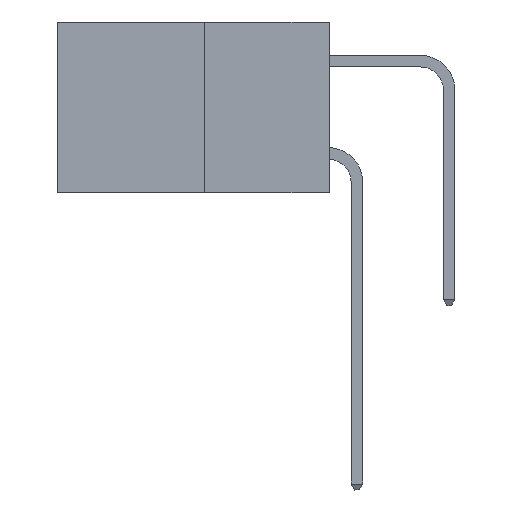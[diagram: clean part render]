
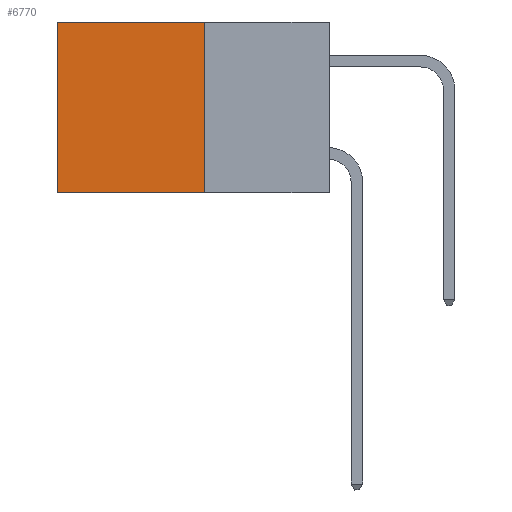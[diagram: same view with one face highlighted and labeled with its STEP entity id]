
A CAD part, left-side view. The second image highlights one B-rep face of the part: STEP entity #6770.
In plain terms, the highlighted planar face has unit normal (-1, 0, 0).
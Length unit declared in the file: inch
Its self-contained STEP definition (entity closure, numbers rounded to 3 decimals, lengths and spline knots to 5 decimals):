
#591 = EDGE_CURVE ( 'NONE', #4315, #26354, #10231, .T. ) ;
#898 = AXIS2_PLACEMENT_3D ( 'NONE', #22842, #24895, #12266 ) ;
#1099 = DIRECTION ( 'NONE',  ( 0., 0., -1. ) ) ;
#3910 = EDGE_CURVE ( 'NONE', #16811, #21445, #14292, .T. ) ;
#4246 = CARTESIAN_POINT ( 'NONE',  ( 0.277, 0.27, -0.37 ) ) ;
#4315 = VERTEX_POINT ( 'NONE', #27012 ) ;
#5430 = CARTESIAN_POINT ( 'NONE',  ( 0.277, 0.59, -0.37 ) ) ;
#6505 = DIRECTION ( 'NONE',  ( 0., 1., 0. ) ) ;
#6594 = DIRECTION ( 'NONE',  ( 0., 1., 0. ) ) ;
#6672 = ORIENTED_EDGE ( 'NONE', *, *, #24980, .F. ) ;
#6735 = CARTESIAN_POINT ( 'NONE',  ( 0.277, 0.27, 0. ) ) ;
#6770 = ADVANCED_FACE ( 'NONE', ( #9208 ), #20752, .F. ) ;
#7145 = LINE ( 'NONE', #4246, #22006 ) ;
#9208 = FACE_OUTER_BOUND ( 'NONE', #26465, .T. ) ;
#10231 = LINE ( 'NONE', #23910, #26320 ) ;
#12266 = DIRECTION ( 'NONE',  ( 0., 0., -1. ) ) ;
#13982 = CARTESIAN_POINT ( 'NONE',  ( 0.277, 0.59, 0. ) ) ;
#14292 = LINE ( 'NONE', #6735, #24802 ) ;
#14384 = LINE ( 'NONE', #5430, #19386 ) ;
#15435 = CARTESIAN_POINT ( 'NONE',  ( 0.277, 0.27, 0. ) ) ;
#16811 = VERTEX_POINT ( 'NONE', #15435 ) ;
#19016 = DIRECTION ( 'NONE',  ( 0., 0., -1. ) ) ;
#19386 = VECTOR ( 'NONE', #1099, 39.37008 ) ;
#19490 = ORIENTED_EDGE ( 'NONE', *, *, #591, .F. ) ;
#20752 = PLANE ( 'NONE',  #898 ) ;
#21023 = ORIENTED_EDGE ( 'NONE', *, *, #24663, .T. ) ;
#21445 = VERTEX_POINT ( 'NONE', #13982 ) ;
#22006 = VECTOR ( 'NONE', #19016, 39.37008 ) ;
#22842 = CARTESIAN_POINT ( 'NONE',  ( 0.277, 0.27, -0.37 ) ) ;
#23910 = CARTESIAN_POINT ( 'NONE',  ( 0.277, 0.27, -0.37 ) ) ;
#24663 = EDGE_CURVE ( 'NONE', #21445, #26354, #14384, .T. ) ;
#24802 = VECTOR ( 'NONE', #6505, 39.37008 ) ;
#24895 = DIRECTION ( 'NONE',  ( 1., 0., 0. ) ) ;
#24980 = EDGE_CURVE ( 'NONE', #16811, #4315, #7145, .T. ) ;
#26320 = VECTOR ( 'NONE', #6594, 39.37008 ) ;
#26354 = VERTEX_POINT ( 'NONE', #26789 ) ;
#26449 = ORIENTED_EDGE ( 'NONE', *, *, #3910, .T. ) ;
#26465 = EDGE_LOOP ( 'NONE', ( #21023, #19490, #6672, #26449 ) ) ;
#26789 = CARTESIAN_POINT ( 'NONE',  ( 0.277, 0.59, -0.37 ) ) ;
#27012 = CARTESIAN_POINT ( 'NONE',  ( 0.277, 0.27, -0.37 ) ) ;
